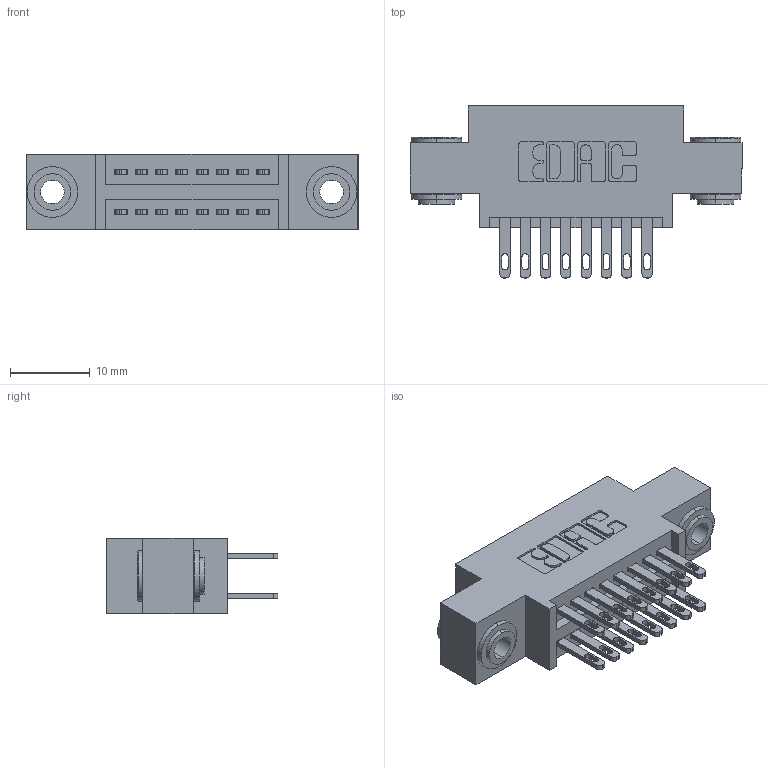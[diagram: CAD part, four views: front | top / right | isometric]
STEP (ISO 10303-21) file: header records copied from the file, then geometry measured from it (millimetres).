
FILE_DESCRIPTION (( 'STEP AP203' ), '1' );
FILE_NAME ('895-016-500-803.STEP', '2020-09-25T04:41:14', ( '' ), ( '' ), 'SwSTEP 2.0', 'SolidWorks 2020', '' );
FILE_SCHEMA (( 'CONFIG_CONTROL_DESIGN' ));
Length unit declared in the file: inch
Products named in the file (4): 345-292-001_345-293-100; 345-250-002_345-250-002-102; 895-016-500-803; 845 Part_0.170 Offset - 0.156 Dia-TH
Assembly tree (19 placements, depth 2):
  895-016-500-803
    845 Part_0.170 Offset - 0.156 Dia-TH
    345-292-001_345-293-100  x16
    345-250-002_345-250-002-102  x2
Bounding box: 41.53 x 21.51 x 9.4 mm (x, y, z)
Volume: 3673.5 mm3; surface area: 5283.1 mm2
Topology: 19 solids, 19 shells, 904 faces, 2685 edges, 1786 vertices
Faces by surface type: plane 526, cylinder 370, cone 8
Entity records: 11566 total; most frequent: CARTESIAN_POINT 1947, ORIENTED_EDGE 1874, DIRECTION 1791, EDGE_CURVE 937, LINE 745, VECTOR 745, VERTEX_POINT 622, AXIS2_PLACEMENT_3D 523
